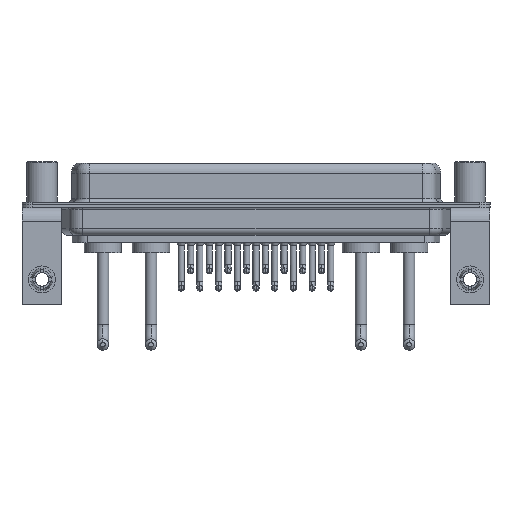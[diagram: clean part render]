
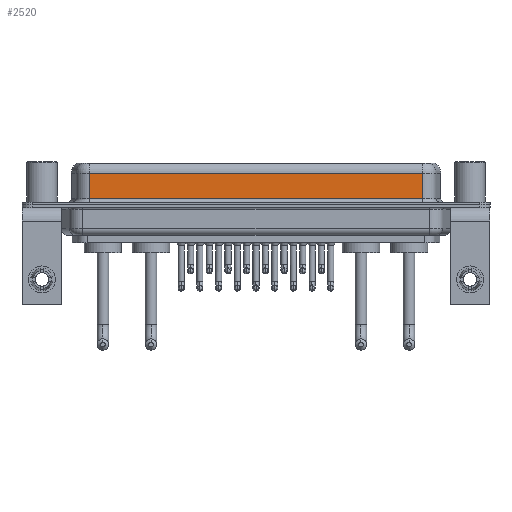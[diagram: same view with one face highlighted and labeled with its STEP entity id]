
A CAD part, front view. The second image highlights one B-rep face of the part: STEP entity #2520.
In plain terms, the highlighted planar face has unit normal (0, -1, 0).
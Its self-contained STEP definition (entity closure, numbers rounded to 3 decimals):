
#888 = LINE ( 'NONE', #8794, #14884 ) ;
#1622 = CARTESIAN_POINT ( 'NONE',  ( 56.462, -3.95, 0.9 ) ) ;
#1708 = CARTESIAN_POINT ( 'NONE',  ( 56.462, -3.95, 0.9 ) ) ;
#1728 = EDGE_LOOP ( 'NONE', ( #7212, #18322, #3427, #23810 ) ) ;
#1817 = CARTESIAN_POINT ( 'NONE',  ( 56.462, -3.95, 4.65 ) ) ;
#2034 = VECTOR ( 'NONE', #21234, 1000. ) ;
#2520 = ADVANCED_FACE ( 'NONE', ( #24771 ), #14967, .F. ) ;
#3222 = VERTEX_POINT ( 'NONE', #1817 ) ;
#3427 = ORIENTED_EDGE ( 'NONE', *, *, #3449, .T. ) ;
#3449 = EDGE_CURVE ( 'NONE', #14699, #19259, #888, .T. ) ;
#4166 = DIRECTION ( 'NONE',  ( 0., 0., -1. ) ) ;
#7212 = ORIENTED_EDGE ( 'NONE', *, *, #25000, .F. ) ;
#7213 = CARTESIAN_POINT ( 'NONE',  ( 56.462, -3.95, 6.4 ) ) ;
#7964 = VECTOR ( 'NONE', #19952, 1000. ) ;
#8794 = CARTESIAN_POINT ( 'NONE',  ( 7.038, -3.95, 6.4 ) ) ;
#12174 = VERTEX_POINT ( 'NONE', #1622 ) ;
#12499 = CARTESIAN_POINT ( 'NONE',  ( 56.462, -3.95, 6.4 ) ) ;
#12887 = DIRECTION ( 'NONE',  ( 0., 0., 1. ) ) ;
#12948 = CARTESIAN_POINT ( 'NONE',  ( 7.038, -3.95, 0.9 ) ) ;
#13598 = VECTOR ( 'NONE', #4166, 1000. ) ;
#13750 = EDGE_CURVE ( 'NONE', #19259, #12174, #21862, .T. ) ;
#14699 = VERTEX_POINT ( 'NONE', #24093 ) ;
#14884 = VECTOR ( 'NONE', #22861, 1000. ) ;
#14967 = PLANE ( 'NONE',  #24250 ) ;
#15090 = DIRECTION ( 'NONE',  ( 0., 1., 0. ) ) ;
#15300 = CARTESIAN_POINT ( 'NONE',  ( 56.462, -3.95, 4.65 ) ) ;
#17242 = LINE ( 'NONE', #15300, #2034 ) ;
#18322 = ORIENTED_EDGE ( 'NONE', *, *, #25271, .T. ) ;
#19259 = VERTEX_POINT ( 'NONE', #12948 ) ;
#19952 = DIRECTION ( 'NONE',  ( 1., 0., 0. ) ) ;
#21234 = DIRECTION ( 'NONE',  ( -1., 0., 0. ) ) ;
#21862 = LINE ( 'NONE', #1708, #7964 ) ;
#22861 = DIRECTION ( 'NONE',  ( 0., 0., -1. ) ) ;
#23810 = ORIENTED_EDGE ( 'NONE', *, *, #13750, .T. ) ;
#24093 = CARTESIAN_POINT ( 'NONE',  ( 7.038, -3.95, 4.65 ) ) ;
#24250 = AXIS2_PLACEMENT_3D ( 'NONE', #12499, #15090, #12887 ) ;
#24771 = FACE_OUTER_BOUND ( 'NONE', #1728, .T. ) ;
#25000 = EDGE_CURVE ( 'NONE', #3222, #12174, #25039, .T. ) ;
#25039 = LINE ( 'NONE', #7213, #13598 ) ;
#25271 = EDGE_CURVE ( 'NONE', #3222, #14699, #17242, .T. ) ;
